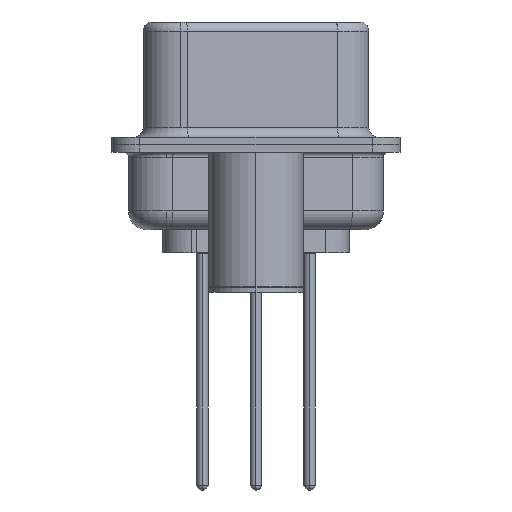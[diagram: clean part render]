
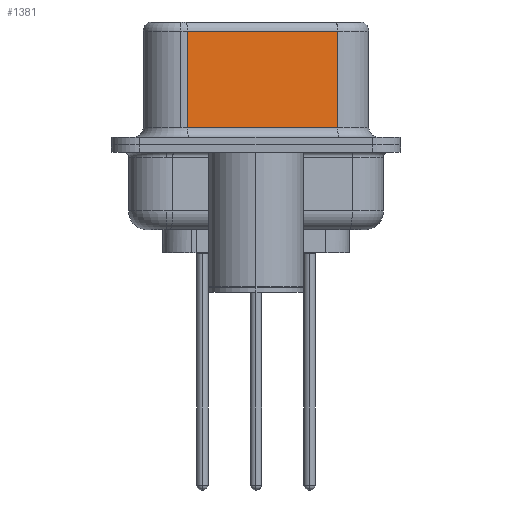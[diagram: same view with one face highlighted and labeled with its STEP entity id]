
A CAD part, left-side view. The second image highlights one B-rep face of the part: STEP entity #1381.
In plain terms, the highlighted planar face has unit normal (-0.985, -0.174, 0).
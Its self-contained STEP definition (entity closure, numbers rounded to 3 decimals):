
#1194 = DIRECTION ( 'NONE',  ( 0.174, -0.985, 0. ) ) ;
#1381 = ADVANCED_FACE ( 'NONE', ( #16938 ), #5366, .F. ) ;
#3223 = ORIENTED_EDGE ( 'NONE', *, *, #21771, .T. ) ;
#4202 = CARTESIAN_POINT ( 'NONE',  ( 5.132, -4.322, 6.02 ) ) ;
#4428 = VERTEX_POINT ( 'NONE', #21713 ) ;
#5366 = PLANE ( 'NONE',  #11171 ) ;
#5519 = DIRECTION ( 'NONE',  ( -0.174, 0.985, 0. ) ) ;
#6342 = CARTESIAN_POINT ( 'NONE',  ( 3.73, 3.628, 6.52 ) ) ;
#7046 = VECTOR ( 'NONE', #20582, 1000. ) ;
#7352 = EDGE_LOOP ( 'NONE', ( #24363, #14794, #3223, #15640 ) ) ;
#9794 = DIRECTION ( 'NONE',  ( 0.985, 0.174, 0. ) ) ;
#10320 = CARTESIAN_POINT ( 'NONE',  ( 3.73, 3.628, 6.02 ) ) ;
#11171 = AXIS2_PLACEMENT_3D ( 'NONE', #11943, #9794, #5519 ) ;
#11462 = DIRECTION ( 'NONE',  ( 0., 0., -1. ) ) ;
#11943 = CARTESIAN_POINT ( 'NONE',  ( 5.132, -4.322, 6.52 ) ) ;
#13741 = LINE ( 'NONE', #16157, #28499 ) ;
#14794 = ORIENTED_EDGE ( 'NONE', *, *, #22438, .T. ) ;
#15486 = VERTEX_POINT ( 'NONE', #18464 ) ;
#15640 = ORIENTED_EDGE ( 'NONE', *, *, #23280, .T. ) ;
#16157 = CARTESIAN_POINT ( 'NONE',  ( 5.132, -4.322, 6.52 ) ) ;
#16214 = VERTEX_POINT ( 'NONE', #10320 ) ;
#16938 = FACE_OUTER_BOUND ( 'NONE', #7352, .T. ) ;
#17867 = CARTESIAN_POINT ( 'NONE',  ( 5.132, -4.322, 6.02 ) ) ;
#17900 = DIRECTION ( 'NONE',  ( 0., 0., -1. ) ) ;
#18464 = CARTESIAN_POINT ( 'NONE',  ( 3.73, 3.628, 0.9 ) ) ;
#19856 = CARTESIAN_POINT ( 'NONE',  ( 5.132, -4.322, 0.9 ) ) ;
#20170 = LINE ( 'NONE', #6342, #22509 ) ;
#20432 = LINE ( 'NONE', #17867, #7046 ) ;
#20582 = DIRECTION ( 'NONE',  ( -0.174, 0.985, 0. ) ) ;
#21713 = CARTESIAN_POINT ( 'NONE',  ( 5.132, -4.322, 0.9 ) ) ;
#21771 = EDGE_CURVE ( 'NONE', #16214, #15486, #20170, .T. ) ;
#21985 = LINE ( 'NONE', #19856, #25953 ) ;
#22330 = VERTEX_POINT ( 'NONE', #4202 ) ;
#22438 = EDGE_CURVE ( 'NONE', #22330, #16214, #20432, .T. ) ;
#22509 = VECTOR ( 'NONE', #17900, 1000. ) ;
#23280 = EDGE_CURVE ( 'NONE', #15486, #4428, #21985, .T. ) ;
#24363 = ORIENTED_EDGE ( 'NONE', *, *, #27114, .F. ) ;
#25953 = VECTOR ( 'NONE', #1194, 1000. ) ;
#27114 = EDGE_CURVE ( 'NONE', #22330, #4428, #13741, .T. ) ;
#28499 = VECTOR ( 'NONE', #11462, 1000. ) ;
